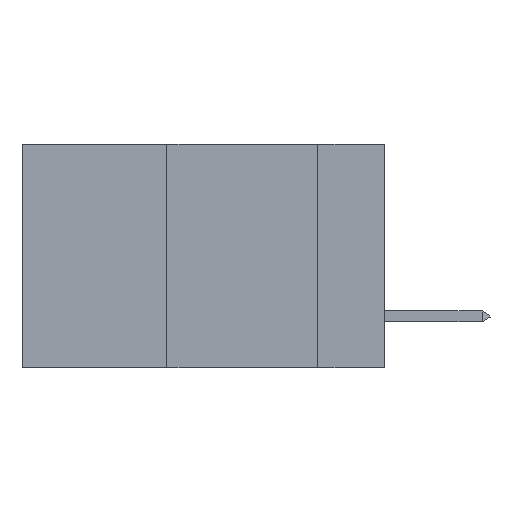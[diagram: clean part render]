
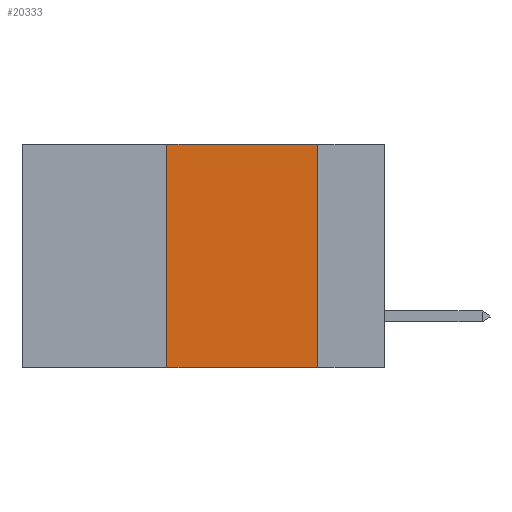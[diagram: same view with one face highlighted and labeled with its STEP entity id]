
A CAD part, left-side view. The second image highlights one B-rep face of the part: STEP entity #20333.
In plain terms, the highlighted planar face has unit normal (-1, 0, 0).
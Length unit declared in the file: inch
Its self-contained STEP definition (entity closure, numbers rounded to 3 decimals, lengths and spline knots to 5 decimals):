
#721 = DIRECTION ( 'NONE',  ( 0., 0., 1. ) ) ;
#2449 = EDGE_CURVE ( 'NONE', #7963, #2734, #31944, .T. ) ;
#2734 = VERTEX_POINT ( 'NONE', #29736 ) ;
#4634 = DIRECTION ( 'NONE',  ( 0., -1., 0. ) ) ;
#5159 = EDGE_CURVE ( 'NONE', #15704, #23670, #35768, .T. ) ;
#5832 = CARTESIAN_POINT ( 'NONE',  ( 0., 0.6, 0. ) ) ;
#6325 = DIRECTION ( 'NONE',  ( 1., 0., 0. ) ) ;
#7692 = AXIS2_PLACEMENT_3D ( 'NONE', #5832, #6325, #36611 ) ;
#7963 = VERTEX_POINT ( 'NONE', #32541 ) ;
#8110 = DIRECTION ( 'NONE',  ( 0., -1., 0. ) ) ;
#8572 = ORIENTED_EDGE ( 'NONE', *, *, #22885, .F. ) ;
#9580 = CARTESIAN_POINT ( 'NONE',  ( 0., 0.11, -0.37 ) ) ;
#10701 = LINE ( 'NONE', #37299, #31999 ) ;
#10997 = CARTESIAN_POINT ( 'NONE',  ( 0., 0.6, -0.37 ) ) ;
#13813 = ORIENTED_EDGE ( 'NONE', *, *, #5159, .F. ) ;
#15285 = ORIENTED_EDGE ( 'NONE', *, *, #2449, .F. ) ;
#15704 = VERTEX_POINT ( 'NONE', #23764 ) ;
#19221 = CARTESIAN_POINT ( 'NONE',  ( 0., 0.11, 0. ) ) ;
#20333 = ADVANCED_FACE ( 'NONE', ( #22075 ), #29884, .F. ) ;
#22075 = FACE_OUTER_BOUND ( 'NONE', #24134, .T. ) ;
#22885 = EDGE_CURVE ( 'NONE', #2734, #15704, #10701, .T. ) ;
#23670 = VERTEX_POINT ( 'NONE', #9580 ) ;
#23764 = CARTESIAN_POINT ( 'NONE',  ( 0., 0.11, 0. ) ) ;
#24134 = EDGE_LOOP ( 'NONE', ( #13813, #8572, #15285, #37894 ) ) ;
#26209 = VECTOR ( 'NONE', #721, 39.37008 ) ;
#28085 = DIRECTION ( 'NONE',  ( 0., 0., -1. ) ) ;
#29736 = CARTESIAN_POINT ( 'NONE',  ( 0., 0.36, 0. ) ) ;
#29884 = PLANE ( 'NONE',  #7692 ) ;
#31944 = LINE ( 'NONE', #37039, #26209 ) ;
#31999 = VECTOR ( 'NONE', #4634, 39.37008 ) ;
#32541 = CARTESIAN_POINT ( 'NONE',  ( 0., 0.36, -0.37 ) ) ;
#32935 = VECTOR ( 'NONE', #28085, 39.37008 ) ;
#33600 = VECTOR ( 'NONE', #8110, 39.37008 ) ;
#35768 = LINE ( 'NONE', #19221, #32935 ) ;
#36033 = EDGE_CURVE ( 'NONE', #7963, #23670, #37394, .T. ) ;
#36611 = DIRECTION ( 'NONE',  ( 0., 0., -1. ) ) ;
#37039 = CARTESIAN_POINT ( 'NONE',  ( 0., 0.36, 0. ) ) ;
#37299 = CARTESIAN_POINT ( 'NONE',  ( 0., 0.6, 0. ) ) ;
#37394 = LINE ( 'NONE', #10997, #33600 ) ;
#37894 = ORIENTED_EDGE ( 'NONE', *, *, #36033, .T. ) ;
